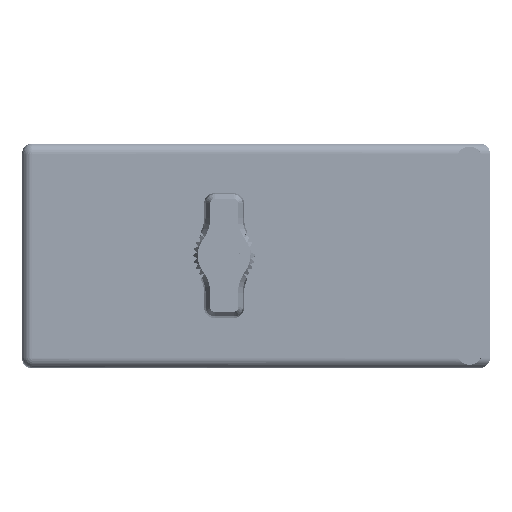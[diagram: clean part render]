
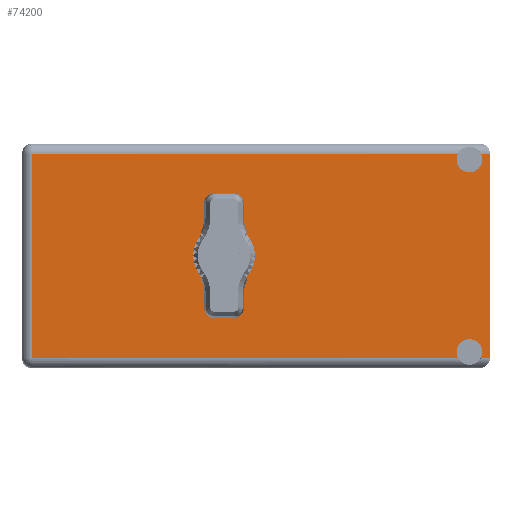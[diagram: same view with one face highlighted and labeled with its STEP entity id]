
A CAD part, top view. The second image highlights one B-rep face of the part: STEP entity #74200.
In plain terms, the highlighted face is planar.
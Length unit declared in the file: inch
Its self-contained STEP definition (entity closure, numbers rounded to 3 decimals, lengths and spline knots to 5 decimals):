
#2062 = DIRECTION ( 'NONE',  ( 0., 0., 1. ) ) ;
#3348 = LINE ( 'NONE', #117401, #62130 ) ;
#6247 = LINE ( 'NONE', #42880, #90956 ) ;
#6493 = ORIENTED_EDGE ( 'NONE', *, *, #82581, .T. ) ;
#7154 = VERTEX_POINT ( 'NONE', #110664 ) ;
#7268 = CARTESIAN_POINT ( 'NONE',  ( 1.3775, 2.03, -0.595 ) ) ;
#7369 = EDGE_CURVE ( 'NONE', #65351, #35091, #3348, .T. ) ;
#7436 = FACE_OUTER_BOUND ( 'NONE', #80446, .T. ) ;
#8777 = EDGE_LOOP ( 'NONE', ( #53503, #23058 ) ) ;
#9748 = EDGE_CURVE ( 'NONE', #36868, #99302, #54642, .T. ) ;
#11540 = ORIENTED_EDGE ( 'NONE', *, *, #40611, .F. ) ;
#13712 = LINE ( 'NONE', #51794, #48063 ) ;
#14203 = CARTESIAN_POINT ( 'NONE',  ( 3.05, 2.03, -0.109 ) ) ;
#14355 = AXIS2_PLACEMENT_3D ( 'NONE', #34848, #17946, #91051 ) ;
#16387 = VERTEX_POINT ( 'NONE', #60326 ) ;
#16967 = VECTOR ( 'NONE', #58286, 39.37008 ) ;
#17946 = DIRECTION ( 'NONE',  ( 0., 1., 0. ) ) ;
#19327 = CARTESIAN_POINT ( 'NONE',  ( 1.3775, 2.03, -0.765 ) ) ;
#21167 = CARTESIAN_POINT ( 'NONE',  ( 3.05, 2.03, -0.109 ) ) ;
#23058 = ORIENTED_EDGE ( 'NONE', *, *, #85931, .F. ) ;
#23808 = DIRECTION ( 'NONE',  ( 0., 1., 0. ) ) ;
#23891 = CARTESIAN_POINT ( 'NONE',  ( 1.3775, 2.03, -0.935 ) ) ;
#24321 = LINE ( 'NONE', #41974, #50013 ) ;
#26763 = CIRCLE ( 'NONE', #110464, 0.17 ) ;
#27814 = PLANE ( 'NONE',  #105770 ) ;
#29296 = CARTESIAN_POINT ( 'NONE',  ( 3.05, 2.03, -1.421 ) ) ;
#30154 = DIRECTION ( 'NONE',  ( 0., 0., 1. ) ) ;
#31111 = CARTESIAN_POINT ( 'NONE',  ( 3.19, 2.03, -1.46 ) ) ;
#33041 = DIRECTION ( 'NONE',  ( 0., 0., 1. ) ) ;
#33157 = CARTESIAN_POINT ( 'NONE',  ( 0.07, 2.03, -0.07 ) ) ;
#33829 = VERTEX_POINT ( 'NONE', #7268 ) ;
#34024 = EDGE_CURVE ( 'NONE', #36868, #7154, #6247, .T. ) ;
#34848 = CARTESIAN_POINT ( 'NONE',  ( 3.05, 2.03, -1.421 ) ) ;
#35091 = VERTEX_POINT ( 'NONE', #60286 ) ;
#35822 = ORIENTED_EDGE ( 'NONE', *, *, #7369, .T. ) ;
#36868 = VERTEX_POINT ( 'NONE', #65706 ) ;
#37054 = CIRCLE ( 'NONE', #14355, 0.0875 ) ;
#40611 = EDGE_CURVE ( 'NONE', #88127, #63197, #105630, .T. ) ;
#40669 = EDGE_CURVE ( 'NONE', #33829, #114153, #83986, .T. ) ;
#41974 = CARTESIAN_POINT ( 'NONE',  ( 0.07, 2.03, -1.53 ) ) ;
#42880 = CARTESIAN_POINT ( 'NONE',  ( 3.19, 2.03, -0.07 ) ) ;
#44353 = EDGE_CURVE ( 'NONE', #35091, #116752, #24321, .T. ) ;
#44983 = EDGE_CURVE ( 'NONE', #104457, #7154, #68711, .T. ) ;
#45294 = ORIENTED_EDGE ( 'NONE', *, *, #76784, .F. ) ;
#46020 = CARTESIAN_POINT ( 'NONE',  ( 0., 2.03, -1.46 ) ) ;
#46059 = CARTESIAN_POINT ( 'NONE',  ( 3.05, 2.03, -0.1965 ) ) ;
#48063 = VECTOR ( 'NONE', #52203, 39.37008 ) ;
#48987 = CARTESIAN_POINT ( 'NONE',  ( 3.19, 2.03, 0. ) ) ;
#49321 = DIRECTION ( 'NONE',  ( 0., 0., 1. ) ) ;
#50013 = VECTOR ( 'NONE', #78119, 39.37008 ) ;
#51233 = CARTESIAN_POINT ( 'NONE',  ( 3.12833, 2.03, -1.46 ) ) ;
#51794 = CARTESIAN_POINT ( 'NONE',  ( 3.19, 2.03, -0.07 ) ) ;
#52203 = DIRECTION ( 'NONE',  ( 1., 0., 0. ) ) ;
#52972 = LINE ( 'NONE', #46020, #80345 ) ;
#53503 = ORIENTED_EDGE ( 'NONE', *, *, #40669, .F. ) ;
#54544 = ORIENTED_EDGE ( 'NONE', *, *, #110491, .F. ) ;
#54642 = CIRCLE ( 'NONE', #94739, 0.0875 ) ;
#57472 = ORIENTED_EDGE ( 'NONE', *, *, #9748, .F. ) ;
#58286 = DIRECTION ( 'NONE',  ( 0., 0., 1. ) ) ;
#60286 = CARTESIAN_POINT ( 'NONE',  ( 0.07, 2.03, -1.46 ) ) ;
#60326 = CARTESIAN_POINT ( 'NONE',  ( 2.97167, 2.03, -0.07 ) ) ;
#62130 = VECTOR ( 'NONE', #62471, 39.37008 ) ;
#62204 = CARTESIAN_POINT ( 'NONE',  ( 3.05, 2.03, -1.3335 ) ) ;
#62471 = DIRECTION ( 'NONE',  ( -1., 0., 0. ) ) ;
#63197 = VERTEX_POINT ( 'NONE', #51233 ) ;
#65351 = VERTEX_POINT ( 'NONE', #115669 ) ;
#65706 = CARTESIAN_POINT ( 'NONE',  ( 3.12833, 2.03, -0.07 ) ) ;
#65976 = DIRECTION ( 'NONE',  ( 0., 1., 0. ) ) ;
#68711 = LINE ( 'NONE', #48987, #16967 ) ;
#71008 = DIRECTION ( 'NONE',  ( 1., 0., 0. ) ) ;
#74200 = ADVANCED_FACE ( 'NONE', ( #102124, #7436 ), #27814, .T. ) ;
#76784 = EDGE_CURVE ( 'NONE', #65351, #88127, #37054, .T. ) ;
#78119 = DIRECTION ( 'NONE',  ( 0., 0., 1. ) ) ;
#80345 = VECTOR ( 'NONE', #81827, 39.37008 ) ;
#80446 = EDGE_LOOP ( 'NONE', ( #115505, #54544, #57472, #99842, #112208, #6493, #11540, #45294, #35822, #87754 ) ) ;
#81827 = DIRECTION ( 'NONE',  ( -1., 0., 0. ) ) ;
#82581 = EDGE_CURVE ( 'NONE', #104457, #63197, #52972, .T. ) ;
#83557 = DIRECTION ( 'NONE',  ( 0., 1., 0. ) ) ;
#83589 = EDGE_CURVE ( 'NONE', #116752, #16387, #13712, .T. ) ;
#83948 = DIRECTION ( 'NONE',  ( 0., 1., 0. ) ) ;
#83986 = CIRCLE ( 'NONE', #86340, 0.17 ) ;
#85424 = DIRECTION ( 'NONE',  ( 0., 1., 0. ) ) ;
#85771 = AXIS2_PLACEMENT_3D ( 'NONE', #21167, #85424, #88616 ) ;
#85931 = EDGE_CURVE ( 'NONE', #114153, #33829, #26763, .T. ) ;
#86340 = AXIS2_PLACEMENT_3D ( 'NONE', #19327, #83557, #49321 ) ;
#86406 = CARTESIAN_POINT ( 'NONE',  ( 1.3775, 2.03, -0.765 ) ) ;
#87754 = ORIENTED_EDGE ( 'NONE', *, *, #44353, .T. ) ;
#88127 = VERTEX_POINT ( 'NONE', #62204 ) ;
#88616 = DIRECTION ( 'NONE',  ( 0., 0., 1. ) ) ;
#90956 = VECTOR ( 'NONE', #71008, 39.37008 ) ;
#91051 = DIRECTION ( 'NONE',  ( 0., 0., 1. ) ) ;
#94739 = AXIS2_PLACEMENT_3D ( 'NONE', #14203, #23808, #33041 ) ;
#95627 = DIRECTION ( 'NONE',  ( 0., 1., 0. ) ) ;
#97066 = AXIS2_PLACEMENT_3D ( 'NONE', #29296, #83948, #2062 ) ;
#99302 = VERTEX_POINT ( 'NONE', #46059 ) ;
#99842 = ORIENTED_EDGE ( 'NONE', *, *, #34024, .T. ) ;
#101302 = CARTESIAN_POINT ( 'NONE',  ( 0., 2.03, -1.53 ) ) ;
#102124 = FACE_BOUND ( 'NONE', #8777, .T. ) ;
#104198 = CIRCLE ( 'NONE', #85771, 0.0875 ) ;
#104457 = VERTEX_POINT ( 'NONE', #31111 ) ;
#105630 = CIRCLE ( 'NONE', #97066, 0.0875 ) ;
#105770 = AXIS2_PLACEMENT_3D ( 'NONE', #101302, #65976, #111258 ) ;
#110464 = AXIS2_PLACEMENT_3D ( 'NONE', #86406, #95627, #30154 ) ;
#110491 = EDGE_CURVE ( 'NONE', #99302, #16387, #104198, .T. ) ;
#110664 = CARTESIAN_POINT ( 'NONE',  ( 3.19, 2.03, -0.07 ) ) ;
#111258 = DIRECTION ( 'NONE',  ( 0., 0., 1. ) ) ;
#112208 = ORIENTED_EDGE ( 'NONE', *, *, #44983, .F. ) ;
#114153 = VERTEX_POINT ( 'NONE', #23891 ) ;
#115505 = ORIENTED_EDGE ( 'NONE', *, *, #83589, .T. ) ;
#115669 = CARTESIAN_POINT ( 'NONE',  ( 2.97167, 2.03, -1.46 ) ) ;
#116752 = VERTEX_POINT ( 'NONE', #33157 ) ;
#117401 = CARTESIAN_POINT ( 'NONE',  ( 0., 2.03, -1.46 ) ) ;
